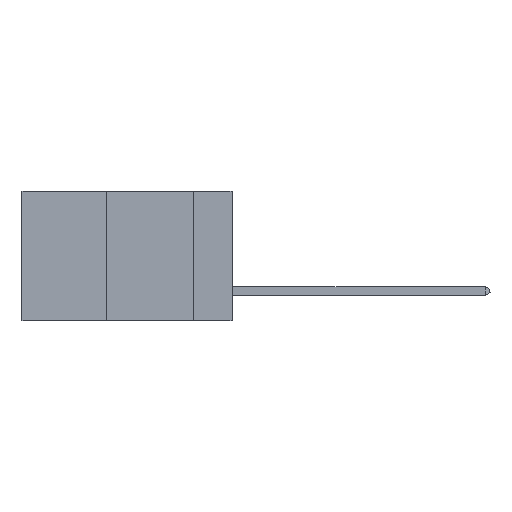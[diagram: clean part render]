
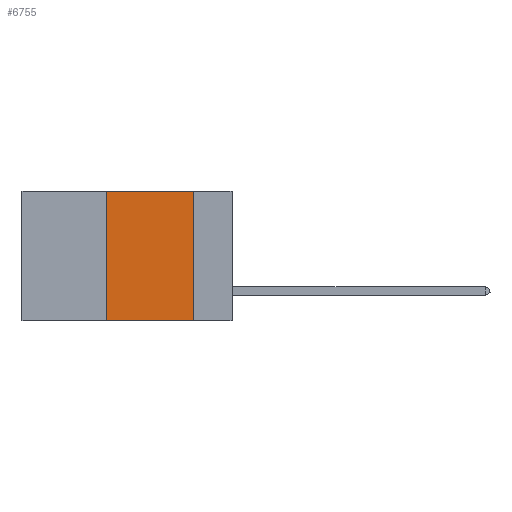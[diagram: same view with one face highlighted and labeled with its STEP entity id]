
A CAD part, left-side view. The second image highlights one B-rep face of the part: STEP entity #6755.
In plain terms, the highlighted planar face has unit normal (-1, 0, 0).
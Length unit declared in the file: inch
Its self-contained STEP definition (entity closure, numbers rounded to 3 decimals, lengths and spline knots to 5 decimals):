
#469 = CARTESIAN_POINT ( 'NONE',  ( 0., 0.6, 0. ) ) ;
#673 = PLANE ( 'NONE',  #8014 ) ;
#943 = LINE ( 'NONE', #2449, #7456 ) ;
#1556 = DIRECTION ( 'NONE',  ( 0., -1., 0. ) ) ;
#1588 = CARTESIAN_POINT ( 'NONE',  ( 0., 0.6, -0.37 ) ) ;
#2214 = VECTOR ( 'NONE', #2265, 39.37008 ) ;
#2265 = DIRECTION ( 'NONE',  ( 0., 0., -1. ) ) ;
#2449 = CARTESIAN_POINT ( 'NONE',  ( 0., 0.36, 0. ) ) ;
#2810 = DIRECTION ( 'NONE',  ( 0., 0., -1. ) ) ;
#2882 = LINE ( 'NONE', #13135, #2214 ) ;
#3640 = CARTESIAN_POINT ( 'NONE',  ( 0., 0.36, 0. ) ) ;
#3918 = CARTESIAN_POINT ( 'NONE',  ( 0., 0.6, 0. ) ) ;
#4141 = EDGE_CURVE ( 'NONE', #4543, #10488, #9989, .T. ) ;
#4377 = VECTOR ( 'NONE', #11347, 39.37008 ) ;
#4457 = ORIENTED_EDGE ( 'NONE', *, *, #10291, .F. ) ;
#4469 = VERTEX_POINT ( 'NONE', #12542 ) ;
#4523 = EDGE_LOOP ( 'NONE', ( #4457, #5131, #10469, #4644 ) ) ;
#4543 = VERTEX_POINT ( 'NONE', #3640 ) ;
#4557 = LINE ( 'NONE', #1588, #4377 ) ;
#4644 = ORIENTED_EDGE ( 'NONE', *, *, #12571, .T. ) ;
#5131 = ORIENTED_EDGE ( 'NONE', *, *, #4141, .F. ) ;
#5632 = VERTEX_POINT ( 'NONE', #9281 ) ;
#5670 = CARTESIAN_POINT ( 'NONE',  ( 0., 0.11, 0. ) ) ;
#6755 = ADVANCED_FACE ( 'NONE', ( #8004 ), #673, .F. ) ;
#7149 = DIRECTION ( 'NONE',  ( 1., 0., 0. ) ) ;
#7456 = VECTOR ( 'NONE', #12240, 39.37008 ) ;
#8004 = FACE_OUTER_BOUND ( 'NONE', #4523, .T. ) ;
#8014 = AXIS2_PLACEMENT_3D ( 'NONE', #3918, #7149, #2810 ) ;
#9281 = CARTESIAN_POINT ( 'NONE',  ( 0., 0.11, -0.37 ) ) ;
#9989 = LINE ( 'NONE', #469, #12037 ) ;
#10291 = EDGE_CURVE ( 'NONE', #10488, #5632, #2882, .T. ) ;
#10469 = ORIENTED_EDGE ( 'NONE', *, *, #12938, .F. ) ;
#10488 = VERTEX_POINT ( 'NONE', #5670 ) ;
#11347 = DIRECTION ( 'NONE',  ( 0., -1., 0. ) ) ;
#12037 = VECTOR ( 'NONE', #1556, 39.37008 ) ;
#12240 = DIRECTION ( 'NONE',  ( 0., 0., 1. ) ) ;
#12542 = CARTESIAN_POINT ( 'NONE',  ( 0., 0.36, -0.37 ) ) ;
#12571 = EDGE_CURVE ( 'NONE', #4469, #5632, #4557, .T. ) ;
#12938 = EDGE_CURVE ( 'NONE', #4469, #4543, #943, .T. ) ;
#13135 = CARTESIAN_POINT ( 'NONE',  ( 0., 0.11, 0. ) ) ;
